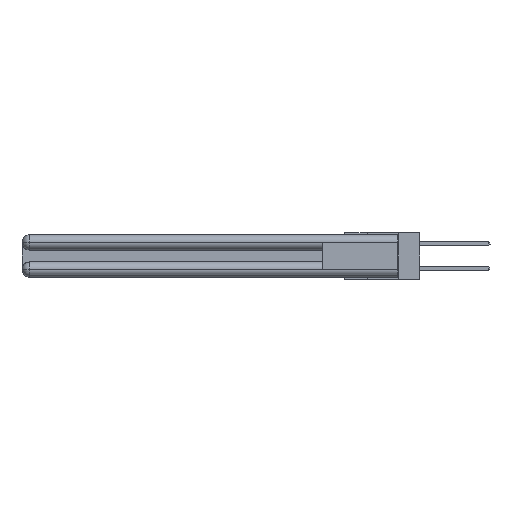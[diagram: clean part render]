
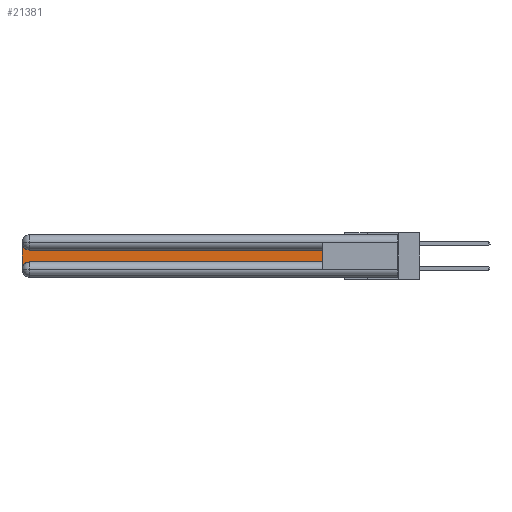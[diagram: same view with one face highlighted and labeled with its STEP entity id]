
A CAD part, left-side view. The second image highlights one B-rep face of the part: STEP entity #21381.
In plain terms, the highlighted planar face has unit normal (-1, 0, 0).
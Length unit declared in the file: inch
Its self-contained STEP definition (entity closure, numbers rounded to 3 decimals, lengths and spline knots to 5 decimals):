
#69 = DIRECTION ( 'NONE',  ( 0., 1., 0. ) ) ;
#161 = VECTOR ( 'NONE', #13671, 39.37008 ) ;
#247 = EDGE_CURVE ( 'NONE', #11498, #16246, #14793, .T. ) ;
#612 = AXIS2_PLACEMENT_3D ( 'NONE', #20093, #29358, #26976 ) ;
#1785 = VERTEX_POINT ( 'NONE', #7447 ) ;
#3505 = EDGE_CURVE ( 'NONE', #26155, #11498, #13394, .T. ) ;
#3883 = DIRECTION ( 'NONE',  ( 0., -1., 0. ) ) ;
#4495 = CARTESIAN_POINT ( 'NONE',  ( 0.075, 3., -0.2775 ) ) ;
#5909 = ORIENTED_EDGE ( 'NONE', *, *, #20157, .T. ) ;
#6739 = VECTOR ( 'NONE', #3883, 39.37008 ) ;
#7447 = CARTESIAN_POINT ( 'NONE',  ( 0.075, 2.94, -0.2175 ) ) ;
#7556 = VECTOR ( 'NONE', #27157, 39.37008 ) ;
#7983 = CARTESIAN_POINT ( 'NONE',  ( 0.075, 2.94, -0.2775 ) ) ;
#8146 = CARTESIAN_POINT ( 'NONE',  ( 0.075, 0.6, -0.1225 ) ) ;
#9110 = CARTESIAN_POINT ( 'NONE',  ( 0.075, 0.6, -0.2175 ) ) ;
#10484 = FACE_OUTER_BOUND ( 'NONE', #16552, .T. ) ;
#11498 = VERTEX_POINT ( 'NONE', #17197 ) ;
#11638 = EDGE_CURVE ( 'NONE', #27023, #26155, #24104, .T. ) ;
#11782 = ORIENTED_EDGE ( 'NONE', *, *, #28096, .T. ) ;
#13394 = LINE ( 'NONE', #22620, #25567 ) ;
#13623 = EDGE_CURVE ( 'NONE', #16246, #23827, #28938, .T. ) ;
#13671 = DIRECTION ( 'NONE',  ( 0., 0., 1. ) ) ;
#13690 = CIRCLE ( 'NONE', #26627, 0.06 ) ;
#14232 = LINE ( 'NONE', #26725, #6739 ) ;
#14793 = CIRCLE ( 'NONE', #612, 0.06 ) ;
#14918 = CARTESIAN_POINT ( 'NONE',  ( 0.075, 0.6, -0.2175 ) ) ;
#15475 = ORIENTED_EDGE ( 'NONE', *, *, #3505, .T. ) ;
#15667 = CARTESIAN_POINT ( 'NONE',  ( 0.075, 3., -0.2175 ) ) ;
#15819 = DIRECTION ( 'NONE',  ( 0., 0., -1. ) ) ;
#16107 = AXIS2_PLACEMENT_3D ( 'NONE', #20147, #24929, #15819 ) ;
#16246 = VERTEX_POINT ( 'NONE', #16616 ) ;
#16552 = EDGE_LOOP ( 'NONE', ( #15475, #23768, #26046, #11782, #5909, #24474 ) ) ;
#16616 = CARTESIAN_POINT ( 'NONE',  ( 0.075, 3., -0.0625 ) ) ;
#17197 = CARTESIAN_POINT ( 'NONE',  ( 0.075, 2.94, -0.1225 ) ) ;
#20093 = CARTESIAN_POINT ( 'NONE',  ( 0.075, 2.94, -0.0625 ) ) ;
#20147 = CARTESIAN_POINT ( 'NONE',  ( 0.075, 3., -0.1225 ) ) ;
#20157 = EDGE_CURVE ( 'NONE', #1785, #27023, #14232, .T. ) ;
#21381 = ADVANCED_FACE ( 'NONE', ( #10484 ), #22537, .F. ) ;
#22537 = PLANE ( 'NONE',  #16107 ) ;
#22620 = CARTESIAN_POINT ( 'NONE',  ( 0.075, 0.6, -0.1225 ) ) ;
#23768 = ORIENTED_EDGE ( 'NONE', *, *, #247, .T. ) ;
#23827 = VERTEX_POINT ( 'NONE', #4495 ) ;
#24104 = LINE ( 'NONE', #9110, #161 ) ;
#24474 = ORIENTED_EDGE ( 'NONE', *, *, #11638, .T. ) ;
#24929 = DIRECTION ( 'NONE',  ( 1., 0., 0. ) ) ;
#25567 = VECTOR ( 'NONE', #69, 39.37008 ) ;
#26046 = ORIENTED_EDGE ( 'NONE', *, *, #13623, .T. ) ;
#26155 = VERTEX_POINT ( 'NONE', #8146 ) ;
#26320 = DIRECTION ( 'NONE',  ( 1., 0., 0. ) ) ;
#26627 = AXIS2_PLACEMENT_3D ( 'NONE', #7983, #26320, #28799 ) ;
#26725 = CARTESIAN_POINT ( 'NONE',  ( 0.075, 0.6, -0.2175 ) ) ;
#26976 = DIRECTION ( 'NONE',  ( 0., 0., -1. ) ) ;
#27023 = VERTEX_POINT ( 'NONE', #14918 ) ;
#27157 = DIRECTION ( 'NONE',  ( 0., 0., -1. ) ) ;
#28096 = EDGE_CURVE ( 'NONE', #23827, #1785, #13690, .T. ) ;
#28799 = DIRECTION ( 'NONE',  ( 0., 0., -1. ) ) ;
#28938 = LINE ( 'NONE', #15667, #7556 ) ;
#29358 = DIRECTION ( 'NONE',  ( 1., 0., 0. ) ) ;
